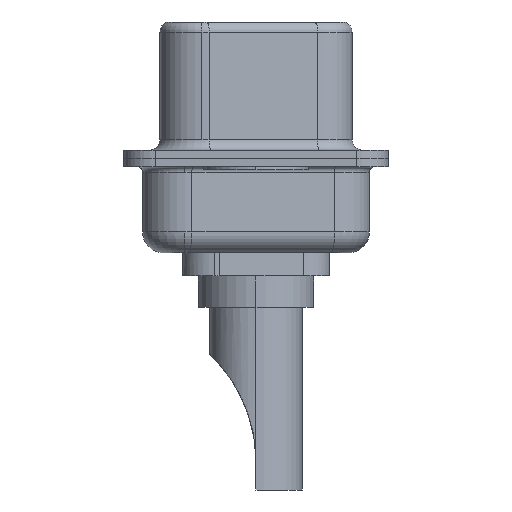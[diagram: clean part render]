
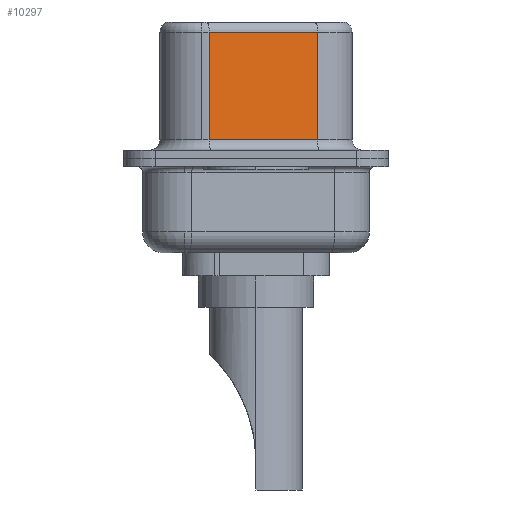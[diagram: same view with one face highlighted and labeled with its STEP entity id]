
A CAD part, left-side view. The second image highlights one B-rep face of the part: STEP entity #10297.
In plain terms, the highlighted planar face has unit normal (-0.985, -0.174, 0).
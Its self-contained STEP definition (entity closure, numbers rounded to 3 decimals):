
#53 = VERTEX_POINT ( 'NONE', #14502 ) ;
#833 = AXIS2_PLACEMENT_3D ( 'NONE', #4213, #2891, #12394 ) ;
#1084 = VERTEX_POINT ( 'NONE', #5982 ) ;
#1900 = CARTESIAN_POINT ( 'NONE',  ( 3.675, 2.233, 6.02 ) ) ;
#2090 = EDGE_CURVE ( 'NONE', #53, #1084, #3676, .T. ) ;
#2119 = ORIENTED_EDGE ( 'NONE', *, *, #11834, .T. ) ;
#2221 = ORIENTED_EDGE ( 'NONE', *, *, #10796, .T. ) ;
#2407 = DIRECTION ( 'NONE',  ( -0.174, 0.985, 0. ) ) ;
#2891 = DIRECTION ( 'NONE',  ( 0.985, 0.174, 0. ) ) ;
#3544 = DIRECTION ( 'NONE',  ( 0., 0., -1. ) ) ;
#3589 = VERTEX_POINT ( 'NONE', #1900 ) ;
#3644 = VECTOR ( 'NONE', #2407, 1000. ) ;
#3676 = LINE ( 'NONE', #14815, #17505 ) ;
#4213 = CARTESIAN_POINT ( 'NONE',  ( 4.585, -2.927, 6.52 ) ) ;
#5982 = CARTESIAN_POINT ( 'NONE',  ( 4.585, -2.927, 0.9 ) ) ;
#6151 = LINE ( 'NONE', #10341, #12540 ) ;
#7722 = EDGE_LOOP ( 'NONE', ( #15513, #2221, #2119, #13594 ) ) ;
#9158 = VECTOR ( 'NONE', #10449, 1000. ) ;
#9579 = CARTESIAN_POINT ( 'NONE',  ( 4.585, -2.927, 6.02 ) ) ;
#10297 = ADVANCED_FACE ( 'NONE', ( #10485 ), #16611, .F. ) ;
#10341 = CARTESIAN_POINT ( 'NONE',  ( 4.585, -2.927, 6.52 ) ) ;
#10400 = CARTESIAN_POINT ( 'NONE',  ( 3.675, 2.233, 6.52 ) ) ;
#10449 = DIRECTION ( 'NONE',  ( 0., 0., -1. ) ) ;
#10485 = FACE_OUTER_BOUND ( 'NONE', #7722, .T. ) ;
#10796 = EDGE_CURVE ( 'NONE', #17708, #3589, #14609, .T. ) ;
#11834 = EDGE_CURVE ( 'NONE', #3589, #53, #12344, .T. ) ;
#12344 = LINE ( 'NONE', #10400, #9158 ) ;
#12394 = DIRECTION ( 'NONE',  ( -0.174, 0.985, 0. ) ) ;
#12540 = VECTOR ( 'NONE', #3544, 1000. ) ;
#12570 = EDGE_CURVE ( 'NONE', #17708, #1084, #6151, .T. ) ;
#12733 = DIRECTION ( 'NONE',  ( 0.174, -0.985, 0. ) ) ;
#13594 = ORIENTED_EDGE ( 'NONE', *, *, #2090, .T. ) ;
#14502 = CARTESIAN_POINT ( 'NONE',  ( 3.675, 2.233, 0.9 ) ) ;
#14609 = LINE ( 'NONE', #14933, #3644 ) ;
#14815 = CARTESIAN_POINT ( 'NONE',  ( 4.585, -2.927, 0.9 ) ) ;
#14933 = CARTESIAN_POINT ( 'NONE',  ( 4.585, -2.927, 6.02 ) ) ;
#15513 = ORIENTED_EDGE ( 'NONE', *, *, #12570, .F. ) ;
#16611 = PLANE ( 'NONE',  #833 ) ;
#17505 = VECTOR ( 'NONE', #12733, 1000. ) ;
#17708 = VERTEX_POINT ( 'NONE', #9579 ) ;
